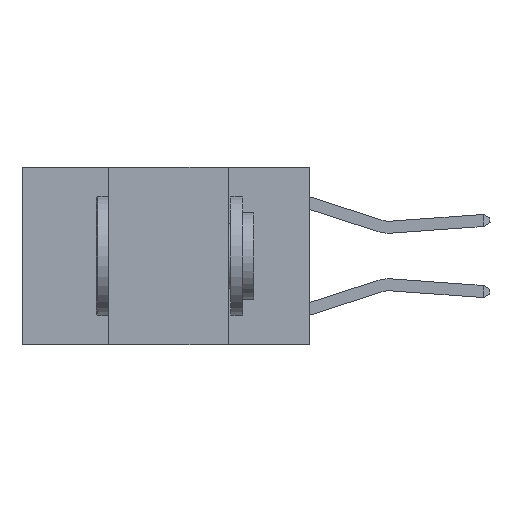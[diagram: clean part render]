
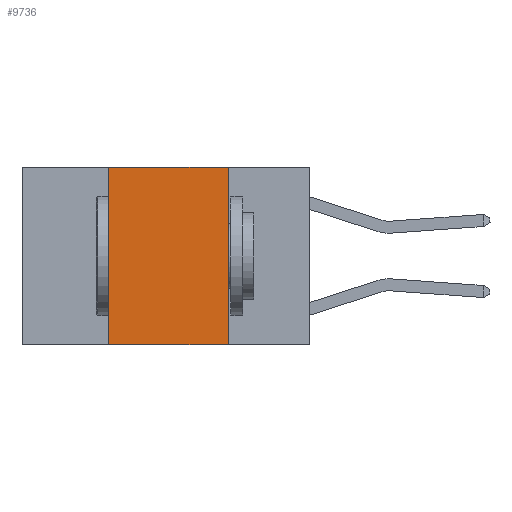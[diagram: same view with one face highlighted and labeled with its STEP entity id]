
A CAD part, left-side view. The second image highlights one B-rep face of the part: STEP entity #9736.
In plain terms, the highlighted planar face has unit normal (-1, 0, 0).
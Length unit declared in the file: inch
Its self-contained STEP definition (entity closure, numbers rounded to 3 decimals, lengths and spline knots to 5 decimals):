
#33 = DIRECTION ( 'NONE',  ( 1., 0., 0. ) ) ;
#718 = VERTEX_POINT ( 'NONE', #6215 ) ;
#1102 = EDGE_CURVE ( 'NONE', #13994, #718, #15482, .T. ) ;
#1573 = AXIS2_PLACEMENT_3D ( 'NONE', #5450, #33, #9418 ) ;
#1586 = ORIENTED_EDGE ( 'NONE', *, *, #1102, .F. ) ;
#2012 = ORIENTED_EDGE ( 'NONE', *, *, #12872, .F. ) ;
#2316 = CARTESIAN_POINT ( 'NONE',  ( 0., 0.42, 0. ) ) ;
#2407 = VECTOR ( 'NONE', #3061, 39.37008 ) ;
#3061 = DIRECTION ( 'NONE',  ( 0., -1., 0. ) ) ;
#4358 = CARTESIAN_POINT ( 'NONE',  ( 0., 0.6, 0. ) ) ;
#4546 = VECTOR ( 'NONE', #4957, 39.37008 ) ;
#4957 = DIRECTION ( 'NONE',  ( 0., 0., 1. ) ) ;
#5276 = EDGE_CURVE ( 'NONE', #6929, #13994, #16146, .T. ) ;
#5450 = CARTESIAN_POINT ( 'NONE',  ( 0., 0.6, 0. ) ) ;
#5962 = CARTESIAN_POINT ( 'NONE',  ( 0., 0.17, 0. ) ) ;
#6057 = FACE_OUTER_BOUND ( 'NONE', #8265, .T. ) ;
#6215 = CARTESIAN_POINT ( 'NONE',  ( 0., 0.17, -0.37 ) ) ;
#6421 = CARTESIAN_POINT ( 'NONE',  ( 0., 0.42, -0.37 ) ) ;
#6788 = PLANE ( 'NONE',  #1573 ) ;
#6801 = EDGE_CURVE ( 'NONE', #8124, #718, #8210, .T. ) ;
#6929 = VERTEX_POINT ( 'NONE', #12832 ) ;
#7232 = DIRECTION ( 'NONE',  ( 0., 0., -1. ) ) ;
#7550 = DIRECTION ( 'NONE',  ( 0., -1., 0. ) ) ;
#7720 = LINE ( 'NONE', #2316, #4546 ) ;
#8124 = VERTEX_POINT ( 'NONE', #6421 ) ;
#8210 = LINE ( 'NONE', #13916, #15344 ) ;
#8265 = EDGE_LOOP ( 'NONE', ( #1586, #15370, #2012, #15768 ) ) ;
#8615 = CARTESIAN_POINT ( 'NONE',  ( 0., 0.17, 0. ) ) ;
#9418 = DIRECTION ( 'NONE',  ( 0., 0., -1. ) ) ;
#9736 = ADVANCED_FACE ( 'NONE', ( #6057 ), #6788, .F. ) ;
#12175 = VECTOR ( 'NONE', #7232, 39.37008 ) ;
#12832 = CARTESIAN_POINT ( 'NONE',  ( 0., 0.42, 0. ) ) ;
#12872 = EDGE_CURVE ( 'NONE', #8124, #6929, #7720, .T. ) ;
#13916 = CARTESIAN_POINT ( 'NONE',  ( 0., 0.6, -0.37 ) ) ;
#13994 = VERTEX_POINT ( 'NONE', #5962 ) ;
#15344 = VECTOR ( 'NONE', #7550, 39.37008 ) ;
#15370 = ORIENTED_EDGE ( 'NONE', *, *, #5276, .F. ) ;
#15482 = LINE ( 'NONE', #8615, #12175 ) ;
#15768 = ORIENTED_EDGE ( 'NONE', *, *, #6801, .T. ) ;
#16146 = LINE ( 'NONE', #4358, #2407 ) ;
